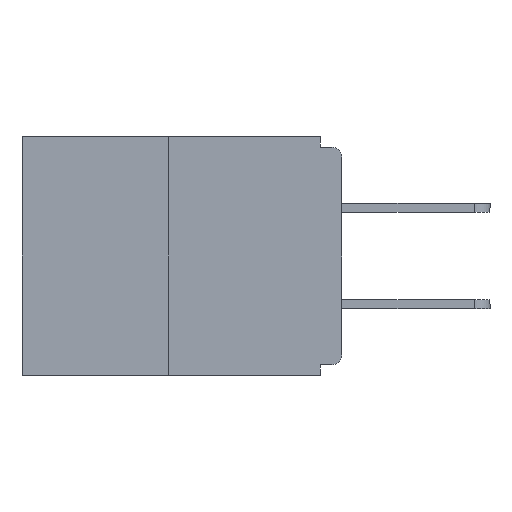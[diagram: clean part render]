
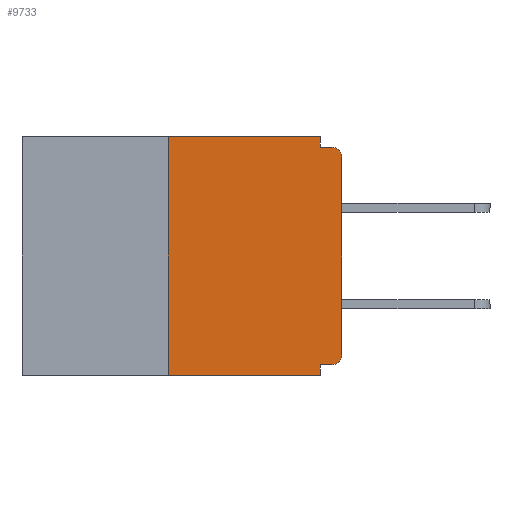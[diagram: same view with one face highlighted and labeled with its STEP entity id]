
A CAD part, left-side view. The second image highlights one B-rep face of the part: STEP entity #9733.
In plain terms, the highlighted planar face has unit normal (-1, 0, 0).
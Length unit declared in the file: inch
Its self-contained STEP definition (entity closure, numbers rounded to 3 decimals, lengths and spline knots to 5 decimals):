
#170 = AXIS2_PLACEMENT_3D ( 'NONE', #9859, #3199, #1623 ) ;
#359 = VERTEX_POINT ( 'NONE', #12290 ) ;
#391 = DIRECTION ( 'NONE',  ( 0., -1., 0. ) ) ;
#637 = ORIENTED_EDGE ( 'NONE', *, *, #3640, .F. ) ;
#648 = EDGE_CURVE ( 'NONE', #1010, #10668, #15892, .T. ) ;
#776 = VERTEX_POINT ( 'NONE', #17106 ) ;
#1010 = VERTEX_POINT ( 'NONE', #3255 ) ;
#1309 = VERTEX_POINT ( 'NONE', #16900 ) ;
#1365 = ORIENTED_EDGE ( 'NONE', *, *, #20523, .F. ) ;
#1623 = DIRECTION ( 'NONE',  ( 0., 0., -1. ) ) ;
#2095 = CARTESIAN_POINT ( 'NONE',  ( 0., 0.031, 0. ) ) ;
#2118 = LINE ( 'NONE', #3176, #19887 ) ;
#2303 = VECTOR ( 'NONE', #10626, 39.37008 ) ;
#2878 = CARTESIAN_POINT ( 'NONE',  ( 0., 0.015, -0.313 ) ) ;
#3133 = EDGE_CURVE ( 'NONE', #4083, #776, #5860, .T. ) ;
#3176 = CARTESIAN_POINT ( 'NONE',  ( 0., 0.25, 0. ) ) ;
#3199 = DIRECTION ( 'NONE',  ( 1., 0., 0. ) ) ;
#3217 = CARTESIAN_POINT ( 'NONE',  ( 0., 0., 0. ) ) ;
#3255 = CARTESIAN_POINT ( 'NONE',  ( 0., 0.25, 0. ) ) ;
#3640 = EDGE_CURVE ( 'NONE', #10668, #4083, #11732, .T. ) ;
#3671 = DIRECTION ( 'NONE',  ( -1., 0., 0. ) ) ;
#3872 = CARTESIAN_POINT ( 'NONE',  ( 0., 0., -0.03 ) ) ;
#3895 = CIRCLE ( 'NONE', #19316, 0.015 ) ;
#4083 = VERTEX_POINT ( 'NONE', #10293 ) ;
#4174 = VERTEX_POINT ( 'NONE', #3872 ) ;
#4729 = LINE ( 'NONE', #15599, #2303 ) ;
#5410 = DIRECTION ( 'NONE',  ( 0., 0., -1. ) ) ;
#5860 = LINE ( 'NONE', #8936, #14451 ) ;
#6235 = CARTESIAN_POINT ( 'NONE',  ( 0., 0.031, 0. ) ) ;
#6411 = DIRECTION ( 'NONE',  ( 0., 0., 1. ) ) ;
#6548 = LINE ( 'NONE', #13476, #15958 ) ;
#7095 = ORIENTED_EDGE ( 'NONE', *, *, #648, .F. ) ;
#7686 = EDGE_CURVE ( 'NONE', #1309, #359, #14772, .T. ) ;
#8007 = CARTESIAN_POINT ( 'NONE',  ( 0., 0.031, -0.343 ) ) ;
#8936 = CARTESIAN_POINT ( 'NONE',  ( 0., 0., -0.015 ) ) ;
#9035 = VECTOR ( 'NONE', #19937, 39.37008 ) ;
#9733 = ADVANCED_FACE ( 'NONE', ( #11466 ), #22025, .F. ) ;
#9859 = CARTESIAN_POINT ( 'NONE',  ( 0., 0.46, 0. ) ) ;
#10293 = CARTESIAN_POINT ( 'NONE',  ( 0., 0.031, -0.015 ) ) ;
#10626 = DIRECTION ( 'NONE',  ( 0., -1., 0. ) ) ;
#10668 = VERTEX_POINT ( 'NONE', #2095 ) ;
#11333 = ORIENTED_EDGE ( 'NONE', *, *, #17523, .T. ) ;
#11424 = VERTEX_POINT ( 'NONE', #14094 ) ;
#11466 = FACE_OUTER_BOUND ( 'NONE', #14850, .T. ) ;
#11549 = DIRECTION ( 'NONE',  ( 0., 0., -1. ) ) ;
#11732 = LINE ( 'NONE', #6235, #9035 ) ;
#12290 = CARTESIAN_POINT ( 'NONE',  ( 0., 0.031, -0.343 ) ) ;
#12547 = CARTESIAN_POINT ( 'NONE',  ( 0., 0.015, -0.03 ) ) ;
#12589 = EDGE_CURVE ( 'NONE', #15091, #359, #4729, .T. ) ;
#12700 = ORIENTED_EDGE ( 'NONE', *, *, #3133, .F. ) ;
#12919 = DIRECTION ( 'NONE',  ( 0., -1., 0. ) ) ;
#12942 = VECTOR ( 'NONE', #12919, 39.37008 ) ;
#12947 = VERTEX_POINT ( 'NONE', #16344 ) ;
#13476 = CARTESIAN_POINT ( 'NONE',  ( 0., 0., -0.328 ) ) ;
#13532 = ORIENTED_EDGE ( 'NONE', *, *, #12589, .T. ) ;
#14094 = CARTESIAN_POINT ( 'NONE',  ( 0., 0., -0.313 ) ) ;
#14451 = VECTOR ( 'NONE', #391, 39.37008 ) ;
#14685 = ORIENTED_EDGE ( 'NONE', *, *, #18460, .T. ) ;
#14772 = LINE ( 'NONE', #8007, #18258 ) ;
#14850 = EDGE_LOOP ( 'NONE', ( #7095, #1365, #13532, #20748, #18153, #14685, #19493, #11333, #12700, #637 ) ) ;
#14884 = DIRECTION ( 'NONE',  ( -1., 0., 0. ) ) ;
#15091 = VERTEX_POINT ( 'NONE', #15263 ) ;
#15184 = DIRECTION ( 'NONE',  ( 0., 1., 0. ) ) ;
#15263 = CARTESIAN_POINT ( 'NONE',  ( 0., 0.25, -0.343 ) ) ;
#15543 = EDGE_CURVE ( 'NONE', #11424, #4174, #21866, .T. ) ;
#15599 = CARTESIAN_POINT ( 'NONE',  ( 0., 0.46, -0.343 ) ) ;
#15892 = LINE ( 'NONE', #21027, #12942 ) ;
#15958 = VECTOR ( 'NONE', #15184, 39.37008 ) ;
#16344 = CARTESIAN_POINT ( 'NONE',  ( 0., 0.015, -0.328 ) ) ;
#16611 = DIRECTION ( 'NONE',  ( 0., 0., -1. ) ) ;
#16900 = CARTESIAN_POINT ( 'NONE',  ( 0., 0.031, -0.328 ) ) ;
#17059 = EDGE_CURVE ( 'NONE', #12947, #1309, #6548, .T. ) ;
#17106 = CARTESIAN_POINT ( 'NONE',  ( 0., 0.015, -0.015 ) ) ;
#17523 = EDGE_CURVE ( 'NONE', #4174, #776, #3895, .T. ) ;
#18019 = AXIS2_PLACEMENT_3D ( 'NONE', #2878, #14884, #16611 ) ;
#18153 = ORIENTED_EDGE ( 'NONE', *, *, #17059, .F. ) ;
#18258 = VECTOR ( 'NONE', #11549, 39.37008 ) ;
#18460 = EDGE_CURVE ( 'NONE', #12947, #11424, #21907, .T. ) ;
#18920 = DIRECTION ( 'NONE',  ( 0., 0., 1. ) ) ;
#19316 = AXIS2_PLACEMENT_3D ( 'NONE', #12547, #3671, #5410 ) ;
#19493 = ORIENTED_EDGE ( 'NONE', *, *, #15543, .T. ) ;
#19887 = VECTOR ( 'NONE', #6411, 39.37008 ) ;
#19937 = DIRECTION ( 'NONE',  ( 0., 0., -1. ) ) ;
#20523 = EDGE_CURVE ( 'NONE', #15091, #1010, #2118, .T. ) ;
#20748 = ORIENTED_EDGE ( 'NONE', *, *, #7686, .F. ) ;
#21027 = CARTESIAN_POINT ( 'NONE',  ( 0., 0.46, 0. ) ) ;
#21614 = VECTOR ( 'NONE', #18920, 39.37008 ) ;
#21866 = LINE ( 'NONE', #3217, #21614 ) ;
#21907 = CIRCLE ( 'NONE', #18019, 0.015 ) ;
#22025 = PLANE ( 'NONE',  #170 ) ;
